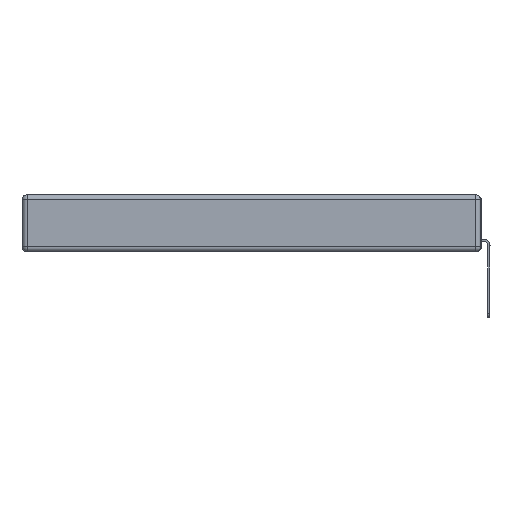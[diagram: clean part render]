
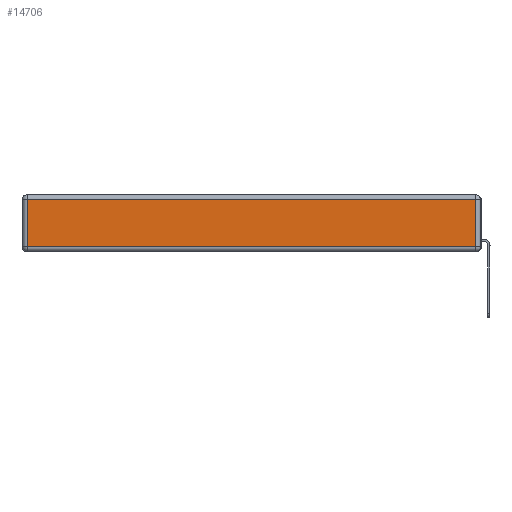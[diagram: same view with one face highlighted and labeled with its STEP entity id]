
A CAD part, left-side view. The second image highlights one B-rep face of the part: STEP entity #14706.
In plain terms, the highlighted planar face has unit normal (-1, 0, 0).
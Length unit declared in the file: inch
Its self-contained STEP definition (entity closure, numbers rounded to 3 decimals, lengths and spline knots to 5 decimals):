
#993 = DIRECTION ( 'NONE',  ( 0., 0., 1. ) ) ;
#1260 = VECTOR ( 'NONE', #11925, 39.37008 ) ;
#1550 = CARTESIAN_POINT ( 'NONE',  ( 0., 0., -0.313 ) ) ;
#2617 = CARTESIAN_POINT ( 'NONE',  ( 0., 0., -0.343 ) ) ;
#2669 = DIRECTION ( 'NONE',  ( 0., -1., 0. ) ) ;
#3061 = LINE ( 'NONE', #6469, #4830 ) ;
#3064 = LINE ( 'NONE', #1550, #7876 ) ;
#4126 = EDGE_CURVE ( 'NONE', #18246, #11456, #17937, .T. ) ;
#4830 = VECTOR ( 'NONE', #12545, 39.37008 ) ;
#5054 = CARTESIAN_POINT ( 'NONE',  ( 0., 2.72, -0.313 ) ) ;
#5551 = CARTESIAN_POINT ( 'NONE',  ( 0., 2.72, -0.343 ) ) ;
#5696 = VERTEX_POINT ( 'NONE', #6753 ) ;
#5784 = ORIENTED_EDGE ( 'NONE', *, *, #4126, .T. ) ;
#6469 = CARTESIAN_POINT ( 'NONE',  ( 0., 0.03, -0.343 ) ) ;
#6753 = CARTESIAN_POINT ( 'NONE',  ( 0., 0.03, -0.03 ) ) ;
#6869 = EDGE_CURVE ( 'NONE', #17502, #5696, #3061, .T. ) ;
#7833 = CARTESIAN_POINT ( 'NONE',  ( 0., 2.75, -0.03 ) ) ;
#7876 = VECTOR ( 'NONE', #2669, 39.37008 ) ;
#8022 = EDGE_CURVE ( 'NONE', #11456, #17502, #3064, .T. ) ;
#8822 = DIRECTION ( 'NONE',  ( -1., 0., 0. ) ) ;
#9650 = ORIENTED_EDGE ( 'NONE', *, *, #13209, .T. ) ;
#10439 = DIRECTION ( 'NONE',  ( 0., 0., -1. ) ) ;
#11456 = VERTEX_POINT ( 'NONE', #5054 ) ;
#11734 = ORIENTED_EDGE ( 'NONE', *, *, #8022, .T. ) ;
#11855 = AXIS2_PLACEMENT_3D ( 'NONE', #2617, #8822, #993 ) ;
#11925 = DIRECTION ( 'NONE',  ( 0., 1., 0. ) ) ;
#11991 = CARTESIAN_POINT ( 'NONE',  ( 0., 0.03, -0.313 ) ) ;
#12545 = DIRECTION ( 'NONE',  ( 0., 0., 1. ) ) ;
#13209 = EDGE_CURVE ( 'NONE', #5696, #18246, #13707, .T. ) ;
#13363 = ORIENTED_EDGE ( 'NONE', *, *, #6869, .T. ) ;
#13707 = LINE ( 'NONE', #7833, #1260 ) ;
#14706 = ADVANCED_FACE ( 'NONE', ( #16287 ), #16382, .T. ) ;
#15649 = CARTESIAN_POINT ( 'NONE',  ( 0., 2.72, -0.03 ) ) ;
#16287 = FACE_OUTER_BOUND ( 'NONE', #16391, .T. ) ;
#16382 = PLANE ( 'NONE',  #11855 ) ;
#16391 = EDGE_LOOP ( 'NONE', ( #11734, #13363, #9650, #5784 ) ) ;
#17502 = VERTEX_POINT ( 'NONE', #11991 ) ;
#17937 = LINE ( 'NONE', #5551, #18323 ) ;
#18246 = VERTEX_POINT ( 'NONE', #15649 ) ;
#18323 = VECTOR ( 'NONE', #10439, 39.37008 ) ;
